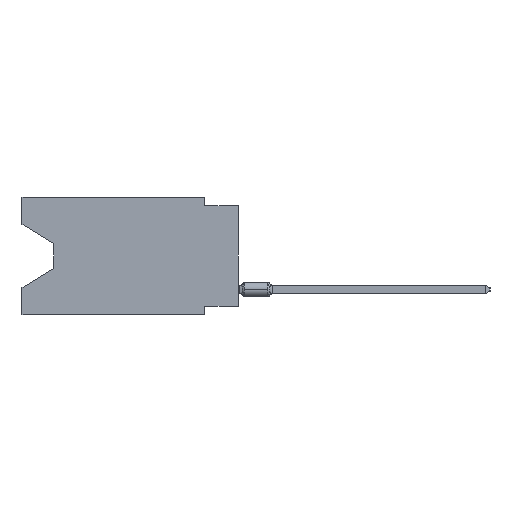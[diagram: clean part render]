
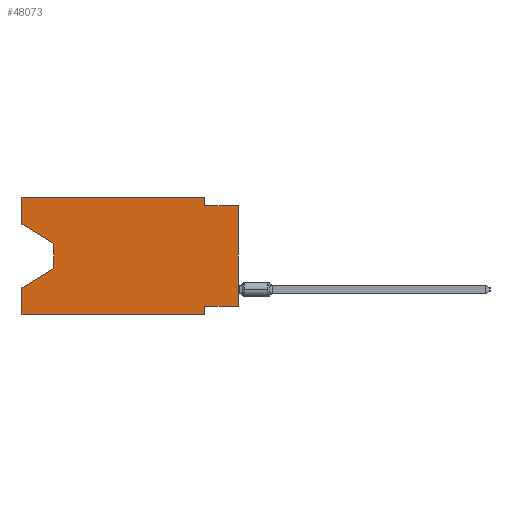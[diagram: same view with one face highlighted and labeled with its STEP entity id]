
A CAD part, left-side view. The second image highlights one B-rep face of the part: STEP entity #48073.
In plain terms, the highlighted planar face has unit normal (-1, 0, 0).
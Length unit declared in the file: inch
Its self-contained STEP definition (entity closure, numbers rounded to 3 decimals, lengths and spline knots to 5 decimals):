
#649 = DIRECTION ( 'NONE',  ( 1., 0., 0. ) ) ;
#853 = EDGE_CURVE ( 'NONE', #51797, #45137, #1976, .T. ) ;
#1559 = LINE ( 'NONE', #37841, #59010 ) ;
#1659 = FACE_OUTER_BOUND ( 'NONE', #40934, .T. ) ;
#1959 = VECTOR ( 'NONE', #57645, 39.37008 ) ;
#1976 = LINE ( 'NONE', #13600, #13251 ) ;
#3199 = ORIENTED_EDGE ( 'NONE', *, *, #18823, .F. ) ;
#4025 = ORIENTED_EDGE ( 'NONE', *, *, #16681, .T. ) ;
#4323 = CARTESIAN_POINT ( 'NONE',  ( 0., 0.55, -0.212 ) ) ;
#5451 = DIRECTION ( 'NONE',  ( 0., 0., -1. ) ) ;
#5921 = ORIENTED_EDGE ( 'NONE', *, *, #853, .F. ) ;
#8068 = CARTESIAN_POINT ( 'NONE',  ( 0., 0.645, -0.35 ) ) ;
#8748 = EDGE_CURVE ( 'NONE', #60431, #11373, #36803, .T. ) ;
#9702 = CARTESIAN_POINT ( 'NONE',  ( 0., 0.1, -0.35 ) ) ;
#10835 = VECTOR ( 'NONE', #46415, 39.37008 ) ;
#11373 = VERTEX_POINT ( 'NONE', #52508 ) ;
#11955 = DIRECTION ( 'NONE',  ( 0., 0., -1. ) ) ;
#12254 = DIRECTION ( 'NONE',  ( 0., 0., 1. ) ) ;
#12613 = CARTESIAN_POINT ( 'NONE',  ( 0., 0.55, -0.138 ) ) ;
#12768 = ORIENTED_EDGE ( 'NONE', *, *, #29178, .F. ) ;
#13005 = CARTESIAN_POINT ( 'NONE',  ( 0., 0.645, -0.35 ) ) ;
#13251 = VECTOR ( 'NONE', #12254, 39.37008 ) ;
#13600 = CARTESIAN_POINT ( 'NONE',  ( 0., 0.645, 0. ) ) ;
#15101 = CARTESIAN_POINT ( 'NONE',  ( 0., 0.55, -0.138 ) ) ;
#15691 = DIRECTION ( 'NONE',  ( 0., 0., 1. ) ) ;
#15728 = VERTEX_POINT ( 'NONE', #24790 ) ;
#16681 = EDGE_CURVE ( 'NONE', #62042, #37258, #55589, .T. ) ;
#18823 = EDGE_CURVE ( 'NONE', #45137, #40830, #36957, .T. ) ;
#19428 = ORIENTED_EDGE ( 'NONE', *, *, #36107, .F. ) ;
#19784 = VECTOR ( 'NONE', #53374, 39.37008 ) ;
#19931 = LINE ( 'NONE', #40789, #43086 ) ;
#20413 = CARTESIAN_POINT ( 'NONE',  ( 0., 0.1, -0.325 ) ) ;
#21108 = CARTESIAN_POINT ( 'NONE',  ( 0., 0.645, 0. ) ) ;
#21174 = CARTESIAN_POINT ( 'NONE',  ( 0., 0.645, 0. ) ) ;
#21234 = LINE ( 'NONE', #62942, #19784 ) ;
#22199 = LINE ( 'NONE', #12613, #60458 ) ;
#23187 = EDGE_CURVE ( 'NONE', #56322, #37258, #50404, .T. ) ;
#24466 = DIRECTION ( 'NONE',  ( 0., -1., 0. ) ) ;
#24790 = CARTESIAN_POINT ( 'NONE',  ( 0., 0., -0.025 ) ) ;
#25131 = ORIENTED_EDGE ( 'NONE', *, *, #26765, .F. ) ;
#25276 = CARTESIAN_POINT ( 'NONE',  ( 0., 0., 0. ) ) ;
#25288 = LINE ( 'NONE', #35549, #35538 ) ;
#26639 = ORIENTED_EDGE ( 'NONE', *, *, #40775, .T. ) ;
#26674 = CARTESIAN_POINT ( 'NONE',  ( 0., 0.645, 0. ) ) ;
#26765 = EDGE_CURVE ( 'NONE', #62042, #11373, #62123, .T. ) ;
#27842 = ORIENTED_EDGE ( 'NONE', *, *, #53666, .T. ) ;
#28264 = ORIENTED_EDGE ( 'NONE', *, *, #23187, .F. ) ;
#28331 = VERTEX_POINT ( 'NONE', #28608 ) ;
#28608 = CARTESIAN_POINT ( 'NONE',  ( 0., 0.1, -0.025 ) ) ;
#29178 = EDGE_CURVE ( 'NONE', #40830, #28331, #21234, .T. ) ;
#30540 = DIRECTION ( 'NONE',  ( 0., 0., -1. ) ) ;
#34019 = VECTOR ( 'NONE', #15691, 39.37008 ) ;
#35538 = VECTOR ( 'NONE', #51278, 39.37008 ) ;
#35549 = CARTESIAN_POINT ( 'NONE',  ( 0., 0., -0.025 ) ) ;
#36107 = EDGE_CURVE ( 'NONE', #28331, #15728, #25288, .T. ) ;
#36803 = LINE ( 'NONE', #4323, #1959 ) ;
#36957 = LINE ( 'NONE', #26674, #43555 ) ;
#37258 = VERTEX_POINT ( 'NONE', #54002 ) ;
#37841 = CARTESIAN_POINT ( 'NONE',  ( 0., 0.645, -0.08025 ) ) ;
#40775 = EDGE_CURVE ( 'NONE', #51797, #63520, #1559, .T. ) ;
#40789 = CARTESIAN_POINT ( 'NONE',  ( 0., 0., -0.325 ) ) ;
#40830 = VERTEX_POINT ( 'NONE', #60010 ) ;
#40934 = EDGE_LOOP ( 'NONE', ( #26639, #49704, #55428, #25131, #4025, #28264, #42204, #27842, #19428, #12768, #3199, #5921 ) ) ;
#41132 = DIRECTION ( 'NONE',  ( 0., 1., 0. ) ) ;
#42204 = ORIENTED_EDGE ( 'NONE', *, *, #59514, .F. ) ;
#42366 = LINE ( 'NONE', #25276, #34019 ) ;
#42398 = VECTOR ( 'NONE', #24466, 39.37008 ) ;
#43086 = VECTOR ( 'NONE', #41132, 39.37008 ) ;
#43555 = VECTOR ( 'NONE', #57795, 39.37008 ) ;
#44909 = VERTEX_POINT ( 'NONE', #67523 ) ;
#45137 = VERTEX_POINT ( 'NONE', #63747 ) ;
#46415 = DIRECTION ( 'NONE',  ( 0., 0., 1. ) ) ;
#48073 = ADVANCED_FACE ( 'NONE', ( #1659 ), #63232, .F. ) ;
#49424 = DIRECTION ( 'NONE',  ( 0., -0.855, -0.519 ) ) ;
#49704 = ORIENTED_EDGE ( 'NONE', *, *, #56031, .T. ) ;
#50404 = LINE ( 'NONE', #9702, #63407 ) ;
#51278 = DIRECTION ( 'NONE',  ( 0., -1., 0. ) ) ;
#51797 = VERTEX_POINT ( 'NONE', #61888 ) ;
#52508 = CARTESIAN_POINT ( 'NONE',  ( 0., 0.645, -0.26975 ) ) ;
#53374 = DIRECTION ( 'NONE',  ( 0., 0., -1. ) ) ;
#53666 = EDGE_CURVE ( 'NONE', #44909, #15728, #42366, .T. ) ;
#54002 = CARTESIAN_POINT ( 'NONE',  ( 0., 0.1, -0.35 ) ) ;
#55428 = ORIENTED_EDGE ( 'NONE', *, *, #8748, .T. ) ;
#55589 = LINE ( 'NONE', #8068, #42398 ) ;
#56031 = EDGE_CURVE ( 'NONE', #63520, #60431, #22199, .T. ) ;
#56322 = VERTEX_POINT ( 'NONE', #20413 ) ;
#57645 = DIRECTION ( 'NONE',  ( 0., 0.855, -0.519 ) ) ;
#57795 = DIRECTION ( 'NONE',  ( 0., -1., 0. ) ) ;
#59010 = VECTOR ( 'NONE', #49424, 39.37008 ) ;
#59514 = EDGE_CURVE ( 'NONE', #44909, #56322, #19931, .T. ) ;
#60010 = CARTESIAN_POINT ( 'NONE',  ( 0., 0.1, 0. ) ) ;
#60431 = VERTEX_POINT ( 'NONE', #60907 ) ;
#60458 = VECTOR ( 'NONE', #11955, 39.37008 ) ;
#60600 = AXIS2_PLACEMENT_3D ( 'NONE', #21174, #649, #5451 ) ;
#60907 = CARTESIAN_POINT ( 'NONE',  ( 0., 0.55, -0.212 ) ) ;
#61888 = CARTESIAN_POINT ( 'NONE',  ( 0., 0.645, -0.08025 ) ) ;
#62042 = VERTEX_POINT ( 'NONE', #13005 ) ;
#62123 = LINE ( 'NONE', #21108, #10835 ) ;
#62942 = CARTESIAN_POINT ( 'NONE',  ( 0., 0.1, 0. ) ) ;
#63232 = PLANE ( 'NONE',  #60600 ) ;
#63407 = VECTOR ( 'NONE', #30540, 39.37008 ) ;
#63520 = VERTEX_POINT ( 'NONE', #15101 ) ;
#63747 = CARTESIAN_POINT ( 'NONE',  ( 0., 0.645, 0. ) ) ;
#67523 = CARTESIAN_POINT ( 'NONE',  ( 0., 0., -0.325 ) ) ;
